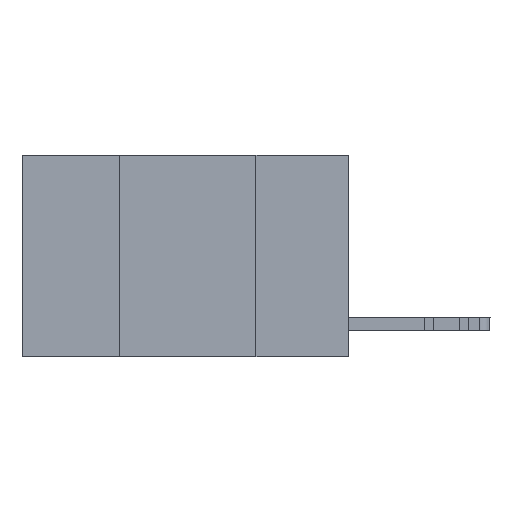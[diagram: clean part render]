
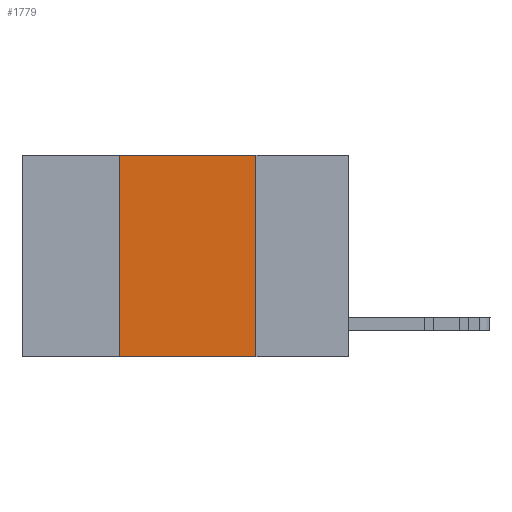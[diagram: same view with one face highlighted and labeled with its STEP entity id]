
A CAD part, left-side view. The second image highlights one B-rep face of the part: STEP entity #1779.
In plain terms, the highlighted planar face has unit normal (-1, 0, 0).
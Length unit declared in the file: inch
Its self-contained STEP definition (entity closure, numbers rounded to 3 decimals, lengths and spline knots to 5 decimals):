
#1340 = LINE ( 'NONE', #25316, #26110 ) ;
#1779 = ADVANCED_FACE ( 'NONE', ( #27335 ), #29250, .F. ) ;
#1834 = CARTESIAN_POINT ( 'NONE',  ( 0., 0.17, 0. ) ) ;
#3371 = LINE ( 'NONE', #22986, #14517 ) ;
#4018 = DIRECTION ( 'NONE',  ( 0., 0., -1. ) ) ;
#4186 = EDGE_LOOP ( 'NONE', ( #19669, #5999, #5046, #24962 ) ) ;
#4397 = DIRECTION ( 'NONE',  ( 0., 0., 1. ) ) ;
#5046 = ORIENTED_EDGE ( 'NONE', *, *, #23916, .F. ) ;
#5872 = CARTESIAN_POINT ( 'NONE',  ( 0., 0.42, 0. ) ) ;
#5999 = ORIENTED_EDGE ( 'NONE', *, *, #25439, .F. ) ;
#7820 = EDGE_CURVE ( 'NONE', #19111, #29995, #18333, .T. ) ;
#12958 = VECTOR ( 'NONE', #29746, 39.37008 ) ;
#13914 = DIRECTION ( 'NONE',  ( 0., -1., 0. ) ) ;
#14377 = VECTOR ( 'NONE', #26763, 39.37008 ) ;
#14517 = VECTOR ( 'NONE', #4397, 39.37008 ) ;
#15086 = LINE ( 'NONE', #28991, #14377 ) ;
#15760 = CARTESIAN_POINT ( 'NONE',  ( 0., 0.6, 0. ) ) ;
#16254 = CARTESIAN_POINT ( 'NONE',  ( 0., 0.6, -0.37 ) ) ;
#18052 = DIRECTION ( 'NONE',  ( 1., 0., 0. ) ) ;
#18333 = LINE ( 'NONE', #16254, #12958 ) ;
#19111 = VERTEX_POINT ( 'NONE', #20557 ) ;
#19669 = ORIENTED_EDGE ( 'NONE', *, *, #27697, .F. ) ;
#20508 = CARTESIAN_POINT ( 'NONE',  ( 0., 0.17, -0.37 ) ) ;
#20557 = CARTESIAN_POINT ( 'NONE',  ( 0., 0.42, -0.37 ) ) ;
#21973 = VERTEX_POINT ( 'NONE', #5872 ) ;
#22986 = CARTESIAN_POINT ( 'NONE',  ( 0., 0.42, 0. ) ) ;
#23908 = VERTEX_POINT ( 'NONE', #1834 ) ;
#23916 = EDGE_CURVE ( 'NONE', #19111, #21973, #3371, .T. ) ;
#24962 = ORIENTED_EDGE ( 'NONE', *, *, #7820, .T. ) ;
#25316 = CARTESIAN_POINT ( 'NONE',  ( 0., 0.6, 0. ) ) ;
#25439 = EDGE_CURVE ( 'NONE', #21973, #23908, #1340, .T. ) ;
#26110 = VECTOR ( 'NONE', #13914, 39.37008 ) ;
#26467 = AXIS2_PLACEMENT_3D ( 'NONE', #15760, #18052, #4018 ) ;
#26763 = DIRECTION ( 'NONE',  ( 0., 0., -1. ) ) ;
#27335 = FACE_OUTER_BOUND ( 'NONE', #4186, .T. ) ;
#27697 = EDGE_CURVE ( 'NONE', #23908, #29995, #15086, .T. ) ;
#28991 = CARTESIAN_POINT ( 'NONE',  ( 0., 0.17, 0. ) ) ;
#29250 = PLANE ( 'NONE',  #26467 ) ;
#29746 = DIRECTION ( 'NONE',  ( 0., -1., 0. ) ) ;
#29995 = VERTEX_POINT ( 'NONE', #20508 ) ;
